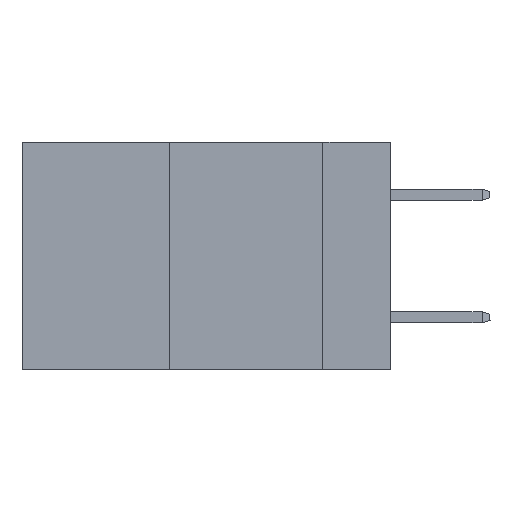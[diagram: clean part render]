
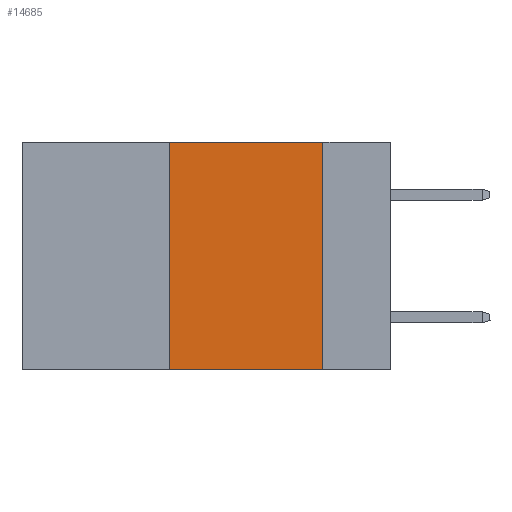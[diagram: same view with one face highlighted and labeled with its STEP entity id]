
A CAD part, left-side view. The second image highlights one B-rep face of the part: STEP entity #14685.
In plain terms, the highlighted planar face has unit normal (-1, 0, 0).
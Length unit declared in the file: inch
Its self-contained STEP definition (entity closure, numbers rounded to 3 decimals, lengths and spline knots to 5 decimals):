
#997 = AXIS2_PLACEMENT_3D ( 'NONE', #4100, #18504, #20483 ) ;
#2461 = ORIENTED_EDGE ( 'NONE', *, *, #10324, .T. ) ;
#3432 = VERTEX_POINT ( 'NONE', #12793 ) ;
#3624 = CARTESIAN_POINT ( 'NONE',  ( 0., 0.36, 0. ) ) ;
#4073 = VERTEX_POINT ( 'NONE', #17395 ) ;
#4100 = CARTESIAN_POINT ( 'NONE',  ( 0., 0.6, 0. ) ) ;
#4872 = CARTESIAN_POINT ( 'NONE',  ( 0., 0.6, -0.37 ) ) ;
#5076 = CARTESIAN_POINT ( 'NONE',  ( 0., 0.11, -0.37 ) ) ;
#5599 = DIRECTION ( 'NONE',  ( 0., 0., 1. ) ) ;
#6342 = LINE ( 'NONE', #4872, #9267 ) ;
#6956 = DIRECTION ( 'NONE',  ( 0., -1., 0. ) ) ;
#7423 = CARTESIAN_POINT ( 'NONE',  ( 0., 0.36, 0. ) ) ;
#8287 = CARTESIAN_POINT ( 'NONE',  ( 0., 0.6, 0. ) ) ;
#8464 = DIRECTION ( 'NONE',  ( 0., -1., 0. ) ) ;
#9267 = VECTOR ( 'NONE', #6956, 39.37008 ) ;
#9637 = FACE_OUTER_BOUND ( 'NONE', #15091, .T. ) ;
#10324 = EDGE_CURVE ( 'NONE', #4073, #17743, #6342, .T. ) ;
#10613 = EDGE_CURVE ( 'NONE', #19697, #3432, #10837, .T. ) ;
#10837 = LINE ( 'NONE', #8287, #24664 ) ;
#11039 = DIRECTION ( 'NONE',  ( 0., 0., -1. ) ) ;
#12067 = LINE ( 'NONE', #21355, #12398 ) ;
#12398 = VECTOR ( 'NONE', #11039, 39.37008 ) ;
#12793 = CARTESIAN_POINT ( 'NONE',  ( 0., 0.11, 0. ) ) ;
#13129 = ORIENTED_EDGE ( 'NONE', *, *, #19632, .F. ) ;
#14668 = ORIENTED_EDGE ( 'NONE', *, *, #10613, .F. ) ;
#14685 = ADVANCED_FACE ( 'NONE', ( #9637 ), #18414, .F. ) ;
#15091 = EDGE_LOOP ( 'NONE', ( #25915, #14668, #13129, #2461 ) ) ;
#17395 = CARTESIAN_POINT ( 'NONE',  ( 0., 0.36, -0.37 ) ) ;
#17743 = VERTEX_POINT ( 'NONE', #5076 ) ;
#18414 = PLANE ( 'NONE',  #997 ) ;
#18504 = DIRECTION ( 'NONE',  ( 1., 0., 0. ) ) ;
#19616 = LINE ( 'NONE', #7423, #20899 ) ;
#19632 = EDGE_CURVE ( 'NONE', #4073, #19697, #19616, .T. ) ;
#19697 = VERTEX_POINT ( 'NONE', #3624 ) ;
#20483 = DIRECTION ( 'NONE',  ( 0., 0., -1. ) ) ;
#20899 = VECTOR ( 'NONE', #5599, 39.37008 ) ;
#21347 = EDGE_CURVE ( 'NONE', #3432, #17743, #12067, .T. ) ;
#21355 = CARTESIAN_POINT ( 'NONE',  ( 0., 0.11, 0. ) ) ;
#24664 = VECTOR ( 'NONE', #8464, 39.37008 ) ;
#25915 = ORIENTED_EDGE ( 'NONE', *, *, #21347, .F. ) ;
